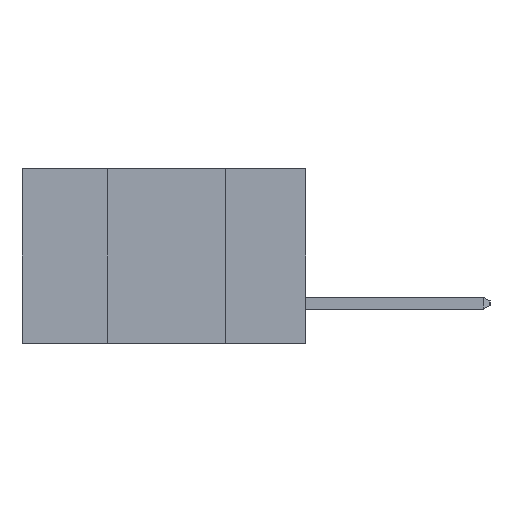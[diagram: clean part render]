
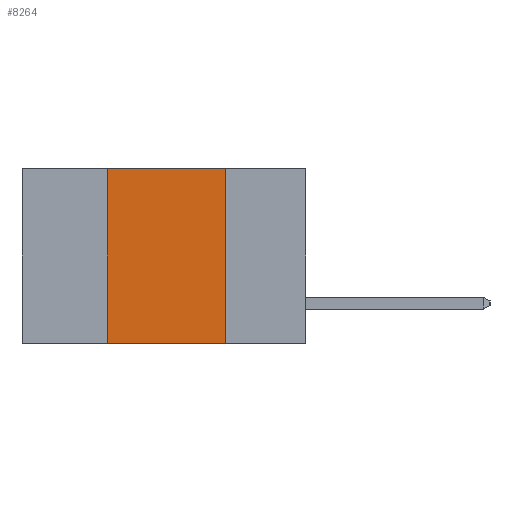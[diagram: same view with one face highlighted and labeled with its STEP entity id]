
A CAD part, left-side view. The second image highlights one B-rep face of the part: STEP entity #8264.
In plain terms, the highlighted planar face has unit normal (-1, 0, 0).
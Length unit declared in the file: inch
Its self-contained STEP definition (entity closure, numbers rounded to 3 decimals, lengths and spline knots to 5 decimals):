
#63 = CARTESIAN_POINT ( 'NONE',  ( 0., 0.6, -0.37 ) ) ;
#524 = EDGE_LOOP ( 'NONE', ( #10971, #10595, #13321, #11103 ) ) ;
#1460 = DIRECTION ( 'NONE',  ( 0., -1., 0. ) ) ;
#1751 = VECTOR ( 'NONE', #1460, 39.37008 ) ;
#2187 = EDGE_CURVE ( 'NONE', #14032, #8863, #12011, .T. ) ;
#3001 = AXIS2_PLACEMENT_3D ( 'NONE', #4392, #14448, #6943 ) ;
#3621 = CARTESIAN_POINT ( 'NONE',  ( 0., 0.17, 0. ) ) ;
#3716 = LINE ( 'NONE', #13059, #5825 ) ;
#4035 = VERTEX_POINT ( 'NONE', #7477 ) ;
#4392 = CARTESIAN_POINT ( 'NONE',  ( 0., 0.6, 0. ) ) ;
#4614 = CARTESIAN_POINT ( 'NONE',  ( 0., 0.17, -0.37 ) ) ;
#5138 = LINE ( 'NONE', #63, #1751 ) ;
#5267 = DIRECTION ( 'NONE',  ( 0., 0., -1. ) ) ;
#5634 = CARTESIAN_POINT ( 'NONE',  ( 0., 0.17, -0.37 ) ) ;
#5825 = VECTOR ( 'NONE', #14271, 39.37008 ) ;
#6943 = DIRECTION ( 'NONE',  ( 0., 0., -1. ) ) ;
#7477 = CARTESIAN_POINT ( 'NONE',  ( 0., 0.42, -0.37 ) ) ;
#8264 = ADVANCED_FACE ( 'NONE', ( #15018 ), #11977, .F. ) ;
#8863 = VERTEX_POINT ( 'NONE', #4614 ) ;
#9167 = EDGE_CURVE ( 'NONE', #4035, #12681, #11215, .T. ) ;
#10595 = ORIENTED_EDGE ( 'NONE', *, *, #16121, .F. ) ;
#10800 = VECTOR ( 'NONE', #16371, 39.37008 ) ;
#10971 = ORIENTED_EDGE ( 'NONE', *, *, #2187, .F. ) ;
#11103 = ORIENTED_EDGE ( 'NONE', *, *, #13003, .T. ) ;
#11215 = LINE ( 'NONE', #15111, #10800 ) ;
#11611 = VECTOR ( 'NONE', #5267, 39.37008 ) ;
#11977 = PLANE ( 'NONE',  #3001 ) ;
#12011 = LINE ( 'NONE', #5634, #11611 ) ;
#12681 = VERTEX_POINT ( 'NONE', #13301 ) ;
#13003 = EDGE_CURVE ( 'NONE', #4035, #8863, #5138, .T. ) ;
#13059 = CARTESIAN_POINT ( 'NONE',  ( 0., 0.6, 0. ) ) ;
#13301 = CARTESIAN_POINT ( 'NONE',  ( 0., 0.42, 0. ) ) ;
#13321 = ORIENTED_EDGE ( 'NONE', *, *, #9167, .F. ) ;
#14032 = VERTEX_POINT ( 'NONE', #3621 ) ;
#14271 = DIRECTION ( 'NONE',  ( 0., -1., 0. ) ) ;
#14448 = DIRECTION ( 'NONE',  ( 1., 0., 0. ) ) ;
#15018 = FACE_OUTER_BOUND ( 'NONE', #524, .T. ) ;
#15111 = CARTESIAN_POINT ( 'NONE',  ( 0., 0.42, -0.37 ) ) ;
#16121 = EDGE_CURVE ( 'NONE', #12681, #14032, #3716, .T. ) ;
#16371 = DIRECTION ( 'NONE',  ( 0., 0., 1. ) ) ;
